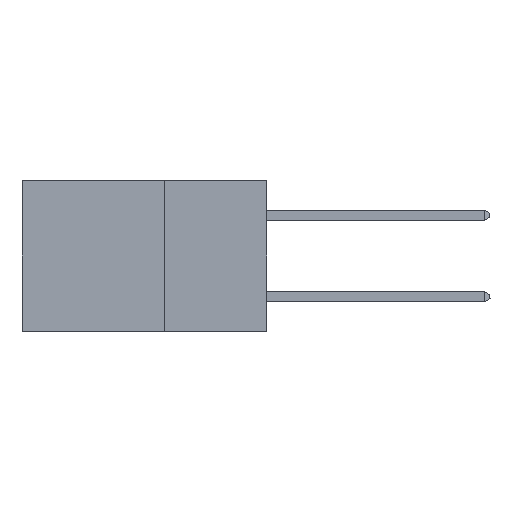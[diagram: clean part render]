
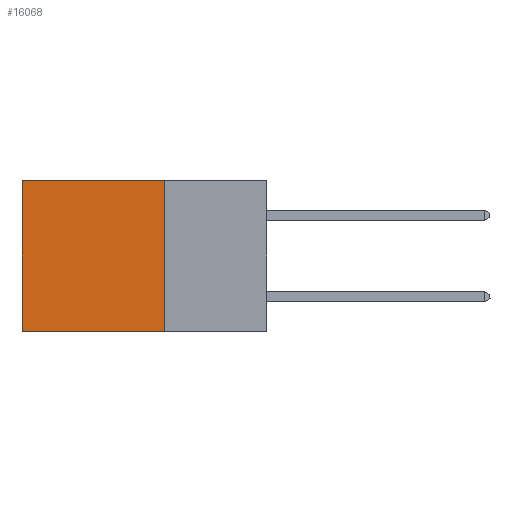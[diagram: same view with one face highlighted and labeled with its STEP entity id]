
A CAD part, left-side view. The second image highlights one B-rep face of the part: STEP entity #16068.
In plain terms, the highlighted planar face has unit normal (-1, 0, 0).
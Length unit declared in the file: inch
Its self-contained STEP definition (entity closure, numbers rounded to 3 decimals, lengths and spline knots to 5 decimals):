
#46 = CARTESIAN_POINT ( 'NONE',  ( 0.2875, 0.25, -0.37 ) ) ;
#159 = VERTEX_POINT ( 'NONE', #46 ) ;
#211 = VECTOR ( 'NONE', #14465, 39.37008 ) ;
#920 = DIRECTION ( 'NONE',  ( 0., 0., -1. ) ) ;
#1444 = VECTOR ( 'NONE', #16357, 39.37008 ) ;
#2096 = PLANE ( 'NONE',  #15970 ) ;
#2601 = EDGE_CURVE ( 'NONE', #9768, #159, #3641, .T. ) ;
#2725 = EDGE_CURVE ( 'NONE', #9768, #11088, #3428, .T. ) ;
#3106 = DIRECTION ( 'NONE',  ( 0., 0., -1. ) ) ;
#3361 = CARTESIAN_POINT ( 'NONE',  ( 0.2875, 0.25, 0. ) ) ;
#3428 = LINE ( 'NONE', #14400, #211 ) ;
#3641 = LINE ( 'NONE', #13474, #6281 ) ;
#3807 = VERTEX_POINT ( 'NONE', #6991 ) ;
#4714 = VECTOR ( 'NONE', #5920, 39.37008 ) ;
#4765 = ORIENTED_EDGE ( 'NONE', *, *, #10434, .T. ) ;
#4803 = CARTESIAN_POINT ( 'NONE',  ( 0.2875, 0.25, 0. ) ) ;
#5382 = EDGE_LOOP ( 'NONE', ( #4765, #7187, #11298, #11832 ) ) ;
#5488 = CARTESIAN_POINT ( 'NONE',  ( 0.2875, 0.6, 0. ) ) ;
#5920 = DIRECTION ( 'NONE',  ( 0., 1., 0. ) ) ;
#6062 = CARTESIAN_POINT ( 'NONE',  ( 0.2875, 0.6, 0. ) ) ;
#6281 = VECTOR ( 'NONE', #3106, 39.37008 ) ;
#6991 = CARTESIAN_POINT ( 'NONE',  ( 0.2875, 0.6, -0.37 ) ) ;
#6997 = DIRECTION ( 'NONE',  ( 1., 0., 0. ) ) ;
#7187 = ORIENTED_EDGE ( 'NONE', *, *, #7455, .F. ) ;
#7455 = EDGE_CURVE ( 'NONE', #159, #3807, #11620, .T. ) ;
#8299 = CARTESIAN_POINT ( 'NONE',  ( 0.2875, 0.25, -0.37 ) ) ;
#9768 = VERTEX_POINT ( 'NONE', #4803 ) ;
#10364 = FACE_OUTER_BOUND ( 'NONE', #5382, .T. ) ;
#10434 = EDGE_CURVE ( 'NONE', #11088, #3807, #14002, .T. ) ;
#11088 = VERTEX_POINT ( 'NONE', #5488 ) ;
#11298 = ORIENTED_EDGE ( 'NONE', *, *, #2601, .F. ) ;
#11620 = LINE ( 'NONE', #8299, #4714 ) ;
#11832 = ORIENTED_EDGE ( 'NONE', *, *, #2725, .T. ) ;
#13474 = CARTESIAN_POINT ( 'NONE',  ( 0.2875, 0.25, 0. ) ) ;
#14002 = LINE ( 'NONE', #6062, #1444 ) ;
#14400 = CARTESIAN_POINT ( 'NONE',  ( 0.2875, 0.25, 0. ) ) ;
#14465 = DIRECTION ( 'NONE',  ( 0., 1., 0. ) ) ;
#15970 = AXIS2_PLACEMENT_3D ( 'NONE', #3361, #6997, #920 ) ;
#16068 = ADVANCED_FACE ( 'NONE', ( #10364 ), #2096, .F. ) ;
#16357 = DIRECTION ( 'NONE',  ( 0., 0., -1. ) ) ;
